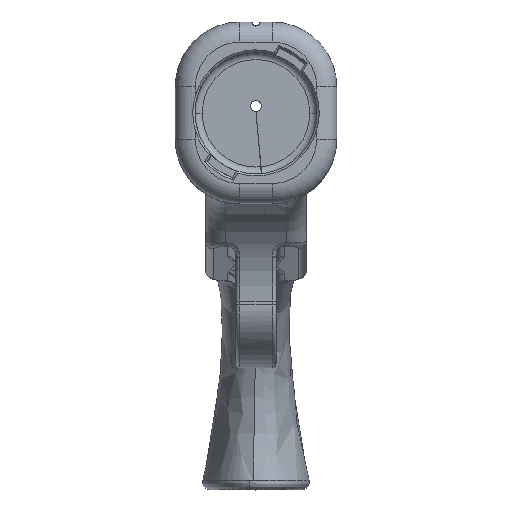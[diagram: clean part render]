
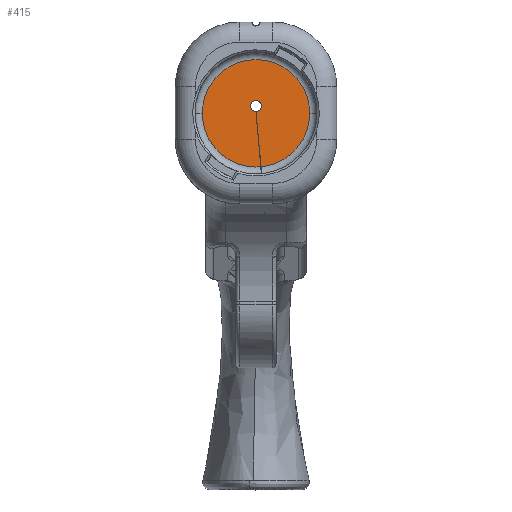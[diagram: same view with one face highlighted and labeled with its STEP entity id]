
A CAD part, top view. The second image highlights one B-rep face of the part: STEP entity #415.
In plain terms, the highlighted planar face has unit normal (0, 0, 1).
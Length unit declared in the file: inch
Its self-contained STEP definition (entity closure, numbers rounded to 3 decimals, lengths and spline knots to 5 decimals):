
#415 = ADVANCED_FACE ( 'NONE', ( #1482, #10415 ), #923, .T. ) ;
#683 = CIRCLE ( 'NONE', #3215, 0.665 ) ;
#923 = PLANE ( 'NONE',  #10473 ) ;
#1157 = EDGE_CURVE ( 'NONE', #10233, #3003, #4013, .T. ) ;
#1482 = FACE_BOUND ( 'NONE', #13205, .T. ) ;
#2149 = DIRECTION ( 'NONE',  ( 1., 0., 0. ) ) ;
#2463 = CARTESIAN_POINT ( 'NONE',  ( 0., 0.09, -3. ) ) ;
#2975 = CARTESIAN_POINT ( 'NONE',  ( -0.07, 0.09, -3. ) ) ;
#3003 = VERTEX_POINT ( 'NONE', #2975 ) ;
#3184 = CIRCLE ( 'NONE', #5721, 0.07 ) ;
#3215 = AXIS2_PLACEMENT_3D ( 'NONE', #5578, #13701, #6739 ) ;
#3332 = EDGE_CURVE ( 'NONE', #5888, #12798, #14842, .T. ) ;
#3623 = DIRECTION ( 'NONE',  ( 1., 0., 0. ) ) ;
#3757 = ORIENTED_EDGE ( 'NONE', *, *, #5576, .F. ) ;
#4013 = CIRCLE ( 'NONE', #4404, 0.07 ) ;
#4404 = AXIS2_PLACEMENT_3D ( 'NONE', #2463, #10608, #3623 ) ;
#4829 = AXIS2_PLACEMENT_3D ( 'NONE', #5363, #13494, #6540 ) ;
#5363 = CARTESIAN_POINT ( 'NONE',  ( 0., 0., -3. ) ) ;
#5576 = EDGE_CURVE ( 'NONE', #3003, #10233, #3184, .T. ) ;
#5578 = CARTESIAN_POINT ( 'NONE',  ( 0., 0., -3. ) ) ;
#5721 = AXIS2_PLACEMENT_3D ( 'NONE', #6762, #14875, #7928 ) ;
#5888 = VERTEX_POINT ( 'NONE', #14614 ) ;
#6540 = DIRECTION ( 'NONE',  ( 1., 0., 0. ) ) ;
#6739 = DIRECTION ( 'NONE',  ( 1., 0., 0. ) ) ;
#6762 = CARTESIAN_POINT ( 'NONE',  ( 0., 0.09, -3. ) ) ;
#7057 = EDGE_LOOP ( 'NONE', ( #11274, #8543 ) ) ;
#7928 = DIRECTION ( 'NONE',  ( 1., 0., 0. ) ) ;
#8543 = ORIENTED_EDGE ( 'NONE', *, *, #13453, .T. ) ;
#9131 = DIRECTION ( 'NONE',  ( 0., 0., 1. ) ) ;
#10233 = VERTEX_POINT ( 'NONE', #11084 ) ;
#10415 = FACE_OUTER_BOUND ( 'NONE', #7057, .T. ) ;
#10473 = AXIS2_PLACEMENT_3D ( 'NONE', #14898, #9131, #2149 ) ;
#10608 = DIRECTION ( 'NONE',  ( 0., 0., 1. ) ) ;
#11084 = CARTESIAN_POINT ( 'NONE',  ( 0.07, 0.09, -3. ) ) ;
#11274 = ORIENTED_EDGE ( 'NONE', *, *, #3332, .T. ) ;
#12798 = VERTEX_POINT ( 'NONE', #13692 ) ;
#13205 = EDGE_LOOP ( 'NONE', ( #3757, #14265 ) ) ;
#13453 = EDGE_CURVE ( 'NONE', #12798, #5888, #683, .T. ) ;
#13494 = DIRECTION ( 'NONE',  ( 0., 0., 1. ) ) ;
#13692 = CARTESIAN_POINT ( 'NONE',  ( -0.665, 0., -3. ) ) ;
#13701 = DIRECTION ( 'NONE',  ( 0., 0., 1. ) ) ;
#14265 = ORIENTED_EDGE ( 'NONE', *, *, #1157, .F. ) ;
#14614 = CARTESIAN_POINT ( 'NONE',  ( 0.665, 0., -3. ) ) ;
#14842 = CIRCLE ( 'NONE', #4829, 0.665 ) ;
#14875 = DIRECTION ( 'NONE',  ( 0., 0., 1. ) ) ;
#14898 = CARTESIAN_POINT ( 'NONE',  ( 0., 0., -3. ) ) ;
